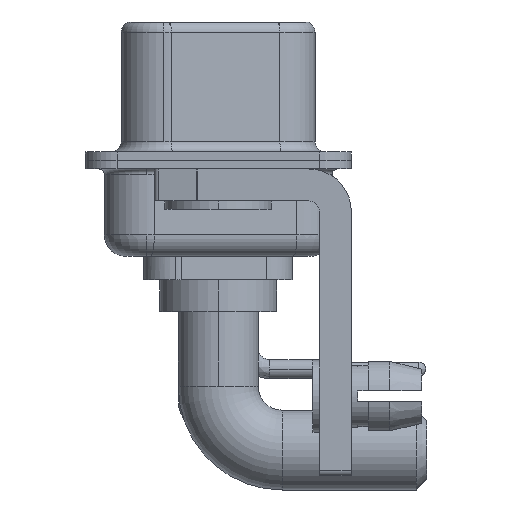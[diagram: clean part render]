
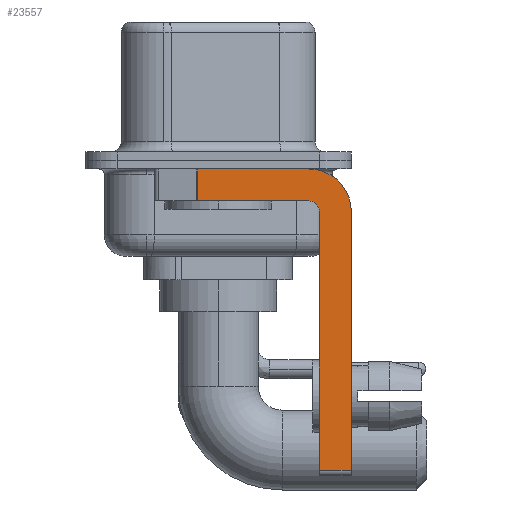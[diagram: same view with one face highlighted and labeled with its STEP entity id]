
A CAD part, left-side view. The second image highlights one B-rep face of the part: STEP entity #23557.
In plain terms, the highlighted planar face has unit normal (-1, 0, 0).
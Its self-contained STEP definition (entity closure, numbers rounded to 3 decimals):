
#550 = EDGE_CURVE ( 'NONE', #4963, #5296, #15631, .T. ) ;
#584 = VECTOR ( 'NONE', #6555, 1000. ) ;
#857 = AXIS2_PLACEMENT_3D ( 'NONE', #8524, #6436, #17675 ) ;
#1731 = VECTOR ( 'NONE', #14480, 1000. ) ;
#2042 = VECTOR ( 'NONE', #13572, 1000. ) ;
#2615 = CIRCLE ( 'NONE', #12552, 0.5 ) ;
#2778 = VERTEX_POINT ( 'NONE', #27608 ) ;
#2784 = ORIENTED_EDGE ( 'NONE', *, *, #3076, .F. ) ;
#2828 = CARTESIAN_POINT ( 'NONE',  ( -2.9, -4.75, -14.55 ) ) ;
#3076 = EDGE_CURVE ( 'NONE', #13437, #2778, #4857, .T. ) ;
#3082 = LINE ( 'NONE', #23619, #1731 ) ;
#3617 = EDGE_CURVE ( 'NONE', #12184, #13437, #2615, .T. ) ;
#3764 = DIRECTION ( 'NONE',  ( 0., 0., -1. ) ) ;
#3881 = ORIENTED_EDGE ( 'NONE', *, *, #18922, .F. ) ;
#4065 = VECTOR ( 'NONE', #5114, 1000. ) ;
#4480 = LINE ( 'NONE', #6123, #584 ) ;
#4857 = LINE ( 'NONE', #22875, #2042 ) ;
#4963 = VERTEX_POINT ( 'NONE', #15939 ) ;
#5114 = DIRECTION ( 'NONE',  ( 0., -1., 0. ) ) ;
#5296 = VERTEX_POINT ( 'NONE', #12411 ) ;
#5613 = ORIENTED_EDGE ( 'NONE', *, *, #19279, .T. ) ;
#5829 = VECTOR ( 'NONE', #15102, 1000. ) ;
#6123 = CARTESIAN_POINT ( 'NONE',  ( -2.9, 0.978, -1.9 ) ) ;
#6303 = FACE_OUTER_BOUND ( 'NONE', #24748, .T. ) ;
#6436 = DIRECTION ( 'NONE',  ( 1., 0., 0. ) ) ;
#6555 = DIRECTION ( 'NONE',  ( 0., 0., -1. ) ) ;
#6943 = CARTESIAN_POINT ( 'NONE',  ( -2.9, -4.75, -2.4 ) ) ;
#7193 = CARTESIAN_POINT ( 'NONE',  ( -2.9, -4.25, -2.4 ) ) ;
#7344 = LINE ( 'NONE', #25325, #4065 ) ;
#7358 = CARTESIAN_POINT ( 'NONE',  ( -2.9, 0.978, -0.4 ) ) ;
#8524 = CARTESIAN_POINT ( 'NONE',  ( -2.9, -4.25, -2.4 ) ) ;
#9164 = ORIENTED_EDGE ( 'NONE', *, *, #3617, .F. ) ;
#9782 = VERTEX_POINT ( 'NONE', #2828 ) ;
#11186 = PLANE ( 'NONE',  #857 ) ;
#12184 = VERTEX_POINT ( 'NONE', #6943 ) ;
#12411 = CARTESIAN_POINT ( 'NONE',  ( -2.9, -6.25, -2.4 ) ) ;
#12552 = AXIS2_PLACEMENT_3D ( 'NONE', #7193, #25190, #20609 ) ;
#12567 = VERTEX_POINT ( 'NONE', #14248 ) ;
#13398 = DIRECTION ( 'NONE',  ( 1., 0., 0. ) ) ;
#13437 = VERTEX_POINT ( 'NONE', #18842 ) ;
#13572 = DIRECTION ( 'NONE',  ( 0., 1., 0. ) ) ;
#14248 = CARTESIAN_POINT ( 'NONE',  ( -2.9, -6.25, -14.55 ) ) ;
#14480 = DIRECTION ( 'NONE',  ( 0., -1., 0. ) ) ;
#15102 = DIRECTION ( 'NONE',  ( 0., 0., 1. ) ) ;
#15631 = CIRCLE ( 'NONE', #18953, 2. ) ;
#15673 = VERTEX_POINT ( 'NONE', #7358 ) ;
#15939 = CARTESIAN_POINT ( 'NONE',  ( -2.9, -4.25, -0.4 ) ) ;
#17675 = DIRECTION ( 'NONE',  ( 0., 0., -1. ) ) ;
#18842 = CARTESIAN_POINT ( 'NONE',  ( -2.9, -4.25, -1.9 ) ) ;
#18843 = LINE ( 'NONE', #20773, #21794 ) ;
#18922 = EDGE_CURVE ( 'NONE', #5296, #12567, #18843, .T. ) ;
#18953 = AXIS2_PLACEMENT_3D ( 'NONE', #24591, #13398, #3764 ) ;
#19279 = EDGE_CURVE ( 'NONE', #15673, #2778, #4480, .T. ) ;
#19854 = EDGE_CURVE ( 'NONE', #9782, #12184, #22184, .T. ) ;
#20609 = DIRECTION ( 'NONE',  ( 0., 0., 1. ) ) ;
#20610 = DIRECTION ( 'NONE',  ( 0., 0., -1. ) ) ;
#20773 = CARTESIAN_POINT ( 'NONE',  ( -2.9, -6.25, -2.4 ) ) ;
#21744 = CARTESIAN_POINT ( 'NONE',  ( -2.9, -4.75, -14.8 ) ) ;
#21794 = VECTOR ( 'NONE', #20610, 1000. ) ;
#21801 = EDGE_CURVE ( 'NONE', #9782, #12567, #7344, .T. ) ;
#22184 = LINE ( 'NONE', #21744, #5829 ) ;
#22566 = ORIENTED_EDGE ( 'NONE', *, *, #19854, .F. ) ;
#22875 = CARTESIAN_POINT ( 'NONE',  ( -2.9, -4.25, -1.9 ) ) ;
#23557 = ADVANCED_FACE ( 'NONE', ( #6303 ), #11186, .F. ) ;
#23619 = CARTESIAN_POINT ( 'NONE',  ( -2.9, 3., -0.4 ) ) ;
#24334 = ORIENTED_EDGE ( 'NONE', *, *, #21801, .T. ) ;
#24591 = CARTESIAN_POINT ( 'NONE',  ( -2.9, -4.25, -2.4 ) ) ;
#24748 = EDGE_LOOP ( 'NONE', ( #26988, #5613, #2784, #9164, #22566, #24334, #3881, #24786 ) ) ;
#24786 = ORIENTED_EDGE ( 'NONE', *, *, #550, .F. ) ;
#25190 = DIRECTION ( 'NONE',  ( -1., 0., 0. ) ) ;
#25325 = CARTESIAN_POINT ( 'NONE',  ( -2.9, -4.25, -14.55 ) ) ;
#26988 = ORIENTED_EDGE ( 'NONE', *, *, #29089, .F. ) ;
#27608 = CARTESIAN_POINT ( 'NONE',  ( -2.9, 0.978, -1.9 ) ) ;
#29089 = EDGE_CURVE ( 'NONE', #15673, #4963, #3082, .T. ) ;
